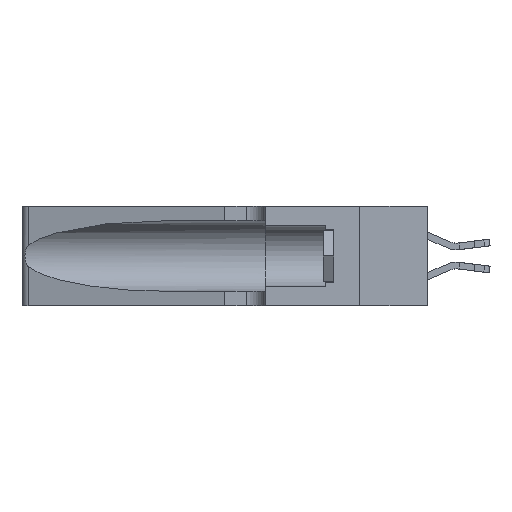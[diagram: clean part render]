
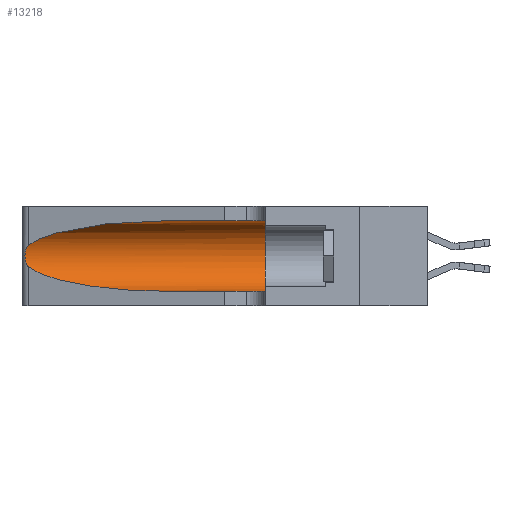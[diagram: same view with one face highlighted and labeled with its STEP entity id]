
A CAD part, left-side view. The second image highlights one B-rep face of the part: STEP entity #13218.
In plain terms, the highlighted cylindrical face has radius 3.308 mm (diameter 6.617 mm), a partial arc.
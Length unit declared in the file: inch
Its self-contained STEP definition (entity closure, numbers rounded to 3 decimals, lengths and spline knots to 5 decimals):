
#285 = CIRCLE ( 'NONE', #19525, 0.13025 ) ;
#302 = CARTESIAN_POINT ( 'NONE',  ( 0.2373, 1.15595, 0.28018 ) ) ;
#848 = ORIENTED_EDGE ( 'NONE', *, *, #4166, .T. ) ;
#935 = EDGE_CURVE ( 'NONE', #11252, #11111, #12536, .T. ) ;
#1020 = CARTESIAN_POINT ( 'NONE',  ( 0.18966, 0.96281, 0.05475 ) ) ;
#1167 = CARTESIAN_POINT ( 'NONE',  ( 0.1305, 0.35, 0.05475 ) ) ;
#1312 = EDGE_CURVE ( 'NONE', #11111, #17246, #285, .T. ) ;
#1361 = CARTESIAN_POINT ( 'NONE',  ( 0.25856, 1.23593, 0.16098 ) ) ;
#1491 = CARTESIAN_POINT ( 'NONE',  ( 0.26017, 1.23833, 0.17102 ) ) ;
#2083 = B_SPLINE_CURVE_WITH_KNOTS ( 'NONE', 3,
 ( #16742, #3028, #10724, #9162, #7470, #9674, #4915, #6081, #1491, #1361, #12232, #7534, #13792, #18231 ),
 .UNSPECIFIED., .F., .F.,
 ( 4, 2, 2, 2, 2, 2, 4 ),
 ( 0., 0.00027, 0.00053, 0.00107, 0.0016, 0.00187, 0.00214 ),
 .UNSPECIFIED. ) ;
#2732 = EDGE_CURVE ( 'NONE', #16532, #7358, #2083, .T. ) ;
#3028 = CARTESIAN_POINT ( 'NONE',  ( 0.25555, 1.22994, 0.2215 ) ) ;
#3057 = FACE_OUTER_BOUND ( 'NONE', #6140, .T. ) ;
#3198 = ORIENTED_EDGE ( 'NONE', *, *, #11280, .T. ) ;
#3428 = ORIENTED_EDGE ( 'NONE', *, *, #2732, .T. ) ;
#4166 = EDGE_CURVE ( 'NONE', #7358, #16464, #13782, .T. ) ;
#4796 = CARTESIAN_POINT ( 'NONE',  ( 0.18966, 0.96281, 0.31525 ) ) ;
#4915 = CARTESIAN_POINT ( 'NONE',  ( 0.26075, 1.23896, 0.19203 ) ) ;
#5386 = CARTESIAN_POINT ( 'NONE',  ( 0.2373, 1.15595, 0.08982 ) ) ;
#5478 = DIRECTION ( 'NONE',  ( 0., -1., 0. ) ) ;
#6081 = CARTESIAN_POINT ( 'NONE',  ( 0.26075, 1.23896, 0.178 ) ) ;
#6140 = EDGE_LOOP ( 'NONE', ( #15652, #3428, #848, #3198, #14446, #17247 ) ) ;
#6409 = CYLINDRICAL_SURFACE ( 'NONE', #7790, 0.13025 ) ;
#6980 = CARTESIAN_POINT ( 'NONE',  ( 0.1305, 0.72297, 0.05475 ) ) ;
#7358 = VERTEX_POINT ( 'NONE', #7405 ) ;
#7405 = CARTESIAN_POINT ( 'NONE',  ( 0.25487, 1.22718, 0.14631 ) ) ;
#7470 = CARTESIAN_POINT ( 'NONE',  ( 0.25854, 1.2359, 0.20912 ) ) ;
#7471 = LINE ( 'NONE', #16348, #9420 ) ;
#7534 = CARTESIAN_POINT ( 'NONE',  ( 0.25639, 1.23186, 0.15144 ) ) ;
#7790 = AXIS2_PLACEMENT_3D ( 'NONE', #14756, #5478, #8636 ) ;
#8636 = DIRECTION ( 'NONE',  ( 0., 0., -1. ) ) ;
#8887 = CARTESIAN_POINT ( 'NONE',  ( 0.1305, 0.72297, 0.05475 ) ) ;
#9162 = CARTESIAN_POINT ( 'NONE',  ( 0.25787, 1.23484, 0.2124 ) ) ;
#9378 = CARTESIAN_POINT ( 'NONE',  ( 0.25487, 1.22718, 0.22369 ) ) ;
#9420 = VECTOR ( 'NONE', #16283, 39.37008 ) ;
#9606 = CARTESIAN_POINT ( 'NONE',  ( 0.1305, 0.35, 0.31525 ) ) ;
#9674 = CARTESIAN_POINT ( 'NONE',  ( 0.26018, 1.23835, 0.19895 ) ) ;
#10289 = DIRECTION ( 'NONE',  ( 0., 0., 1. ) ) ;
#10724 = CARTESIAN_POINT ( 'NONE',  ( 0.25639, 1.23184, 0.21858 ) ) ;
#11111 = VERTEX_POINT ( 'NONE', #9606 ) ;
#11252 = VERTEX_POINT ( 'NONE', #17723 ) ;
#11280 = EDGE_CURVE ( 'NONE', #16464, #17246, #7471, .T. ) ;
#11675 = DIRECTION ( 'NONE',  ( 0., 1., 0. ) ) ;
#11734 = DIRECTION ( 'NONE',  ( 0., -1., 0. ) ) ;
#12232 = CARTESIAN_POINT ( 'NONE',  ( 0.25789, 1.23486, 0.15765 ) ) ;
#12536 = LINE ( 'NONE', #13071, #17338 ) ;
#13071 = CARTESIAN_POINT ( 'NONE',  ( 0.1305, 1.61858, 0.31525 ) ) ;
#13218 = ADVANCED_FACE ( 'NONE', ( #3057 ), #6409, .F. ) ;
#13313 = EDGE_CURVE ( 'NONE', #11252, #16532, #13418, .T. ) ;
#13418 =( BOUNDED_CURVE ( )  B_SPLINE_CURVE ( 3, ( #13993, #4796, #302, #9378 ),
 .UNSPECIFIED., .F., .T. ) 
 B_SPLINE_CURVE_WITH_KNOTS ( ( 4, 4 ),
 ( 1.5708, 2.84003 ),
 .UNSPECIFIED. ) 
 CURVE ( )  GEOMETRIC_REPRESENTATION_ITEM ( )  RATIONAL_B_SPLINE_CURVE ( ( 1., 0.87, 0.87, 1. ) ) 
 REPRESENTATION_ITEM ( '' )  );
#13782 =( BOUNDED_CURVE ( )  B_SPLINE_CURVE ( 3, ( #16177, #5386, #1020, #6980 ),
 .UNSPECIFIED., .F., .F. ) 
 B_SPLINE_CURVE_WITH_KNOTS ( ( 4, 4 ),
 ( 3.44316, 4.71239 ),
 .UNSPECIFIED. ) 
 CURVE ( )  GEOMETRIC_REPRESENTATION_ITEM ( )  RATIONAL_B_SPLINE_CURVE ( ( 1., 0.87, 0.87, 1. ) ) 
 REPRESENTATION_ITEM ( '' )  );
#13792 = CARTESIAN_POINT ( 'NONE',  ( 0.25555, 1.22993, 0.14849 ) ) ;
#13993 = CARTESIAN_POINT ( 'NONE',  ( 0.1305, 0.72297, 0.31525 ) ) ;
#14446 = ORIENTED_EDGE ( 'NONE', *, *, #1312, .F. ) ;
#14516 = CARTESIAN_POINT ( 'NONE',  ( 0.1305, 0.35, 0.185 ) ) ;
#14756 = CARTESIAN_POINT ( 'NONE',  ( 0.1305, 1.61858, 0.185 ) ) ;
#15652 = ORIENTED_EDGE ( 'NONE', *, *, #13313, .T. ) ;
#16177 = CARTESIAN_POINT ( 'NONE',  ( 0.25487, 1.22718, 0.14631 ) ) ;
#16283 = DIRECTION ( 'NONE',  ( 0., -1., 0. ) ) ;
#16348 = CARTESIAN_POINT ( 'NONE',  ( 0.1305, 1.61858, 0.05475 ) ) ;
#16464 = VERTEX_POINT ( 'NONE', #8887 ) ;
#16532 = VERTEX_POINT ( 'NONE', #17353 ) ;
#16742 = CARTESIAN_POINT ( 'NONE',  ( 0.25487, 1.22718, 0.22369 ) ) ;
#17246 = VERTEX_POINT ( 'NONE', #1167 ) ;
#17247 = ORIENTED_EDGE ( 'NONE', *, *, #935, .F. ) ;
#17338 = VECTOR ( 'NONE', #11734, 39.37008 ) ;
#17353 = CARTESIAN_POINT ( 'NONE',  ( 0.25487, 1.22718, 0.22369 ) ) ;
#17723 = CARTESIAN_POINT ( 'NONE',  ( 0.1305, 0.72297, 0.31525 ) ) ;
#18231 = CARTESIAN_POINT ( 'NONE',  ( 0.25487, 1.22718, 0.14631 ) ) ;
#19525 = AXIS2_PLACEMENT_3D ( 'NONE', #14516, #11675, #10289 ) ;
